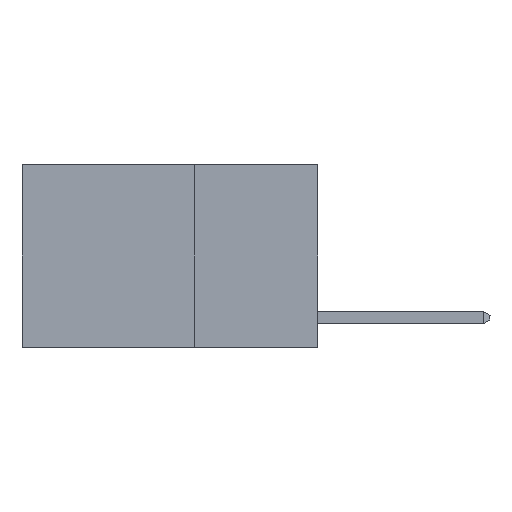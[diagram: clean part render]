
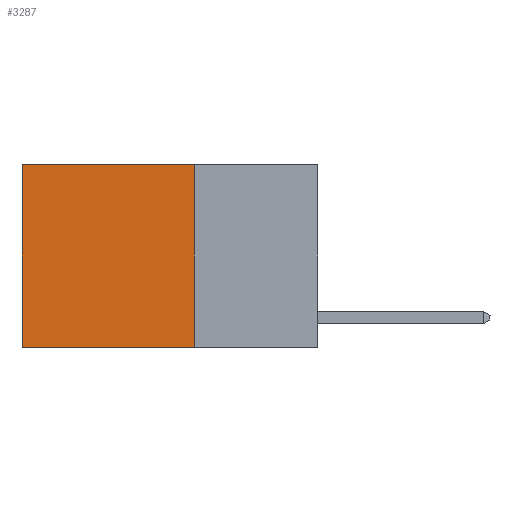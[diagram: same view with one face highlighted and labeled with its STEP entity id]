
A CAD part, left-side view. The second image highlights one B-rep face of the part: STEP entity #3287.
In plain terms, the highlighted planar face has unit normal (-1, 0, 0).
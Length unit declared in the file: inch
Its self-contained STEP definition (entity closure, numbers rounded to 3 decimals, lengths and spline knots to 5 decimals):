
#39 = EDGE_CURVE ( 'NONE', #8913, #10178, #6383, .T. ) ;
#584 = CARTESIAN_POINT ( 'NONE',  ( 0.2625, 0.25, -0.37 ) ) ;
#1051 = CARTESIAN_POINT ( 'NONE',  ( 0.2625, 0.25, 0. ) ) ;
#1204 = DIRECTION ( 'NONE',  ( 0., 0., -1. ) ) ;
#1559 = ORIENTED_EDGE ( 'NONE', *, *, #4140, .T. ) ;
#1642 = VECTOR ( 'NONE', #4949, 39.37008 ) ;
#1804 = AXIS2_PLACEMENT_3D ( 'NONE', #9022, #10830, #5331 ) ;
#2330 = DIRECTION ( 'NONE',  ( 0., 0., -1. ) ) ;
#2762 = FACE_OUTER_BOUND ( 'NONE', #3892, .T. ) ;
#2879 = VERTEX_POINT ( 'NONE', #4612 ) ;
#3287 = ADVANCED_FACE ( 'NONE', ( #2762 ), #9949, .F. ) ;
#3892 = EDGE_LOOP ( 'NONE', ( #5858, #4776, #8908, #1559 ) ) ;
#4140 = EDGE_CURVE ( 'NONE', #2879, #9586, #5880, .T. ) ;
#4612 = CARTESIAN_POINT ( 'NONE',  ( 0.2625, 0.25, 0. ) ) ;
#4776 = ORIENTED_EDGE ( 'NONE', *, *, #39, .F. ) ;
#4949 = DIRECTION ( 'NONE',  ( 0., 1., 0. ) ) ;
#5331 = DIRECTION ( 'NONE',  ( 0., 0., -1. ) ) ;
#5582 = VECTOR ( 'NONE', #10400, 39.37008 ) ;
#5858 = ORIENTED_EDGE ( 'NONE', *, *, #8445, .T. ) ;
#5880 = LINE ( 'NONE', #1051, #5582 ) ;
#5993 = CARTESIAN_POINT ( 'NONE',  ( 0.2625, 0.25, 0. ) ) ;
#6383 = LINE ( 'NONE', #584, #1642 ) ;
#7807 = CARTESIAN_POINT ( 'NONE',  ( 0.2625, 0.6, -0.37 ) ) ;
#7824 = CARTESIAN_POINT ( 'NONE',  ( 0.2625, 0.6, 0. ) ) ;
#7958 = CARTESIAN_POINT ( 'NONE',  ( 0.2625, 0.6, 0. ) ) ;
#8401 = VECTOR ( 'NONE', #2330, 39.37008 ) ;
#8445 = EDGE_CURVE ( 'NONE', #9586, #10178, #10802, .T. ) ;
#8908 = ORIENTED_EDGE ( 'NONE', *, *, #9606, .F. ) ;
#8913 = VERTEX_POINT ( 'NONE', #9604 ) ;
#9022 = CARTESIAN_POINT ( 'NONE',  ( 0.2625, 0.25, 0. ) ) ;
#9586 = VERTEX_POINT ( 'NONE', #7824 ) ;
#9604 = CARTESIAN_POINT ( 'NONE',  ( 0.2625, 0.25, -0.37 ) ) ;
#9606 = EDGE_CURVE ( 'NONE', #2879, #8913, #9935, .T. ) ;
#9935 = LINE ( 'NONE', #5993, #10216 ) ;
#9949 = PLANE ( 'NONE',  #1804 ) ;
#10178 = VERTEX_POINT ( 'NONE', #7807 ) ;
#10216 = VECTOR ( 'NONE', #1204, 39.37008 ) ;
#10400 = DIRECTION ( 'NONE',  ( 0., 1., 0. ) ) ;
#10802 = LINE ( 'NONE', #7958, #8401 ) ;
#10830 = DIRECTION ( 'NONE',  ( 1., 0., 0. ) ) ;
